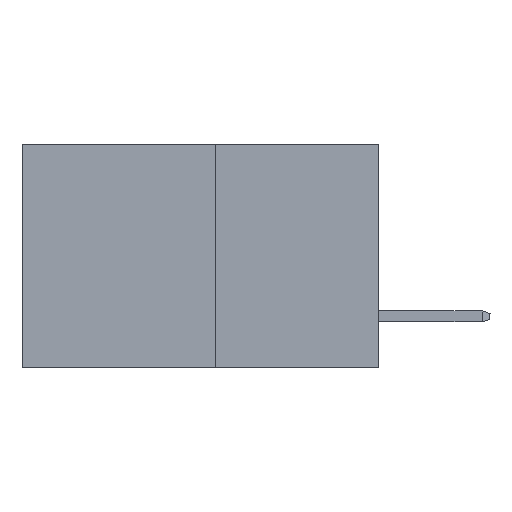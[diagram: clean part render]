
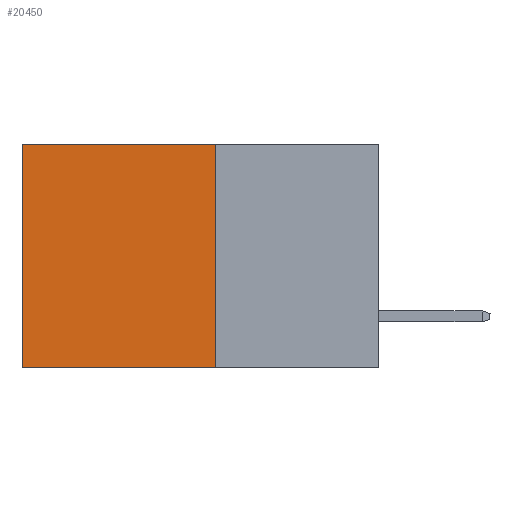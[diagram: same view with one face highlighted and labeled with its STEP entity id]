
A CAD part, left-side view. The second image highlights one B-rep face of the part: STEP entity #20450.
In plain terms, the highlighted planar face has unit normal (-1, 0, 0).
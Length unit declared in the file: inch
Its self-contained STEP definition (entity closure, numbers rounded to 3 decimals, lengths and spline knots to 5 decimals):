
#385 = DIRECTION ( 'NONE',  ( 0., 0., -1. ) ) ;
#800 = CARTESIAN_POINT ( 'NONE',  ( 0.277, 0.27, -0.37 ) ) ;
#2427 = EDGE_CURVE ( 'NONE', #6773, #4105, #3846, .T. ) ;
#3846 = LINE ( 'NONE', #800, #7672 ) ;
#4105 = VERTEX_POINT ( 'NONE', #13570 ) ;
#4346 = VECTOR ( 'NONE', #15603, 39.37008 ) ;
#4938 = DIRECTION ( 'NONE',  ( 0., 1., 0. ) ) ;
#5026 = CARTESIAN_POINT ( 'NONE',  ( 0.277, 0.27, -0.37 ) ) ;
#6215 = PLANE ( 'NONE',  #19830 ) ;
#6287 = DIRECTION ( 'NONE',  ( 0., 0., -1. ) ) ;
#6773 = VERTEX_POINT ( 'NONE', #5026 ) ;
#7402 = EDGE_CURVE ( 'NONE', #19592, #20016, #9695, .T. ) ;
#7672 = VECTOR ( 'NONE', #4938, 39.37008 ) ;
#8031 = VECTOR ( 'NONE', #385, 39.37008 ) ;
#8245 = ORIENTED_EDGE ( 'NONE', *, *, #7402, .T. ) ;
#8824 = DIRECTION ( 'NONE',  ( 0., 0., -1. ) ) ;
#9695 = LINE ( 'NONE', #15580, #4346 ) ;
#10152 = CARTESIAN_POINT ( 'NONE',  ( 0.277, 0.59, -0.37 ) ) ;
#10575 = CARTESIAN_POINT ( 'NONE',  ( 0.277, 0.27, 0. ) ) ;
#10748 = EDGE_CURVE ( 'NONE', #20016, #4105, #16542, .T. ) ;
#10757 = ORIENTED_EDGE ( 'NONE', *, *, #2427, .F. ) ;
#11496 = ORIENTED_EDGE ( 'NONE', *, *, #10748, .T. ) ;
#11566 = VECTOR ( 'NONE', #8824, 39.37008 ) ;
#11752 = CARTESIAN_POINT ( 'NONE',  ( 0.277, 0.59, 0. ) ) ;
#12311 = EDGE_LOOP ( 'NONE', ( #11496, #10757, #13282, #8245 ) ) ;
#12369 = FACE_OUTER_BOUND ( 'NONE', #12311, .T. ) ;
#12717 = CARTESIAN_POINT ( 'NONE',  ( 0.277, 0.27, -0.37 ) ) ;
#13282 = ORIENTED_EDGE ( 'NONE', *, *, #14454, .F. ) ;
#13570 = CARTESIAN_POINT ( 'NONE',  ( 0.277, 0.59, -0.37 ) ) ;
#14454 = EDGE_CURVE ( 'NONE', #19592, #6773, #20005, .T. ) ;
#15580 = CARTESIAN_POINT ( 'NONE',  ( 0.277, 0.27, 0. ) ) ;
#15603 = DIRECTION ( 'NONE',  ( 0., 1., 0. ) ) ;
#15890 = DIRECTION ( 'NONE',  ( 1., 0., 0. ) ) ;
#16542 = LINE ( 'NONE', #10152, #8031 ) ;
#19592 = VERTEX_POINT ( 'NONE', #10575 ) ;
#19830 = AXIS2_PLACEMENT_3D ( 'NONE', #12717, #15890, #6287 ) ;
#19957 = CARTESIAN_POINT ( 'NONE',  ( 0.277, 0.27, -0.37 ) ) ;
#20005 = LINE ( 'NONE', #19957, #11566 ) ;
#20016 = VERTEX_POINT ( 'NONE', #11752 ) ;
#20450 = ADVANCED_FACE ( 'NONE', ( #12369 ), #6215, .F. ) ;
